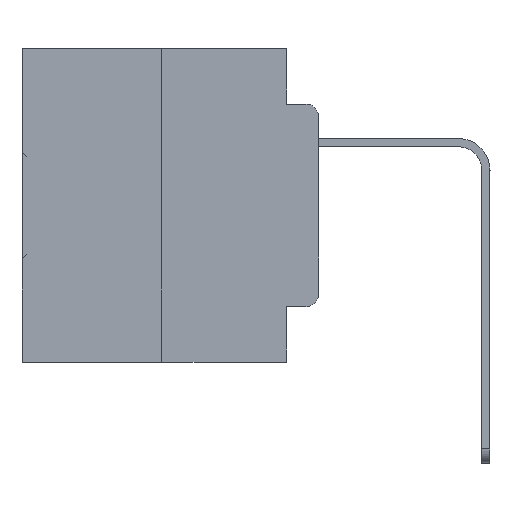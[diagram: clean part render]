
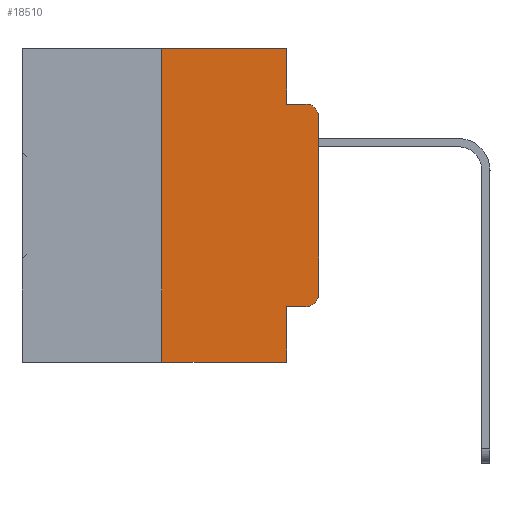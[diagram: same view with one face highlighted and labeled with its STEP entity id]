
A CAD part, left-side view. The second image highlights one B-rep face of the part: STEP entity #18510.
In plain terms, the highlighted planar face has unit normal (-1, 0, 0).
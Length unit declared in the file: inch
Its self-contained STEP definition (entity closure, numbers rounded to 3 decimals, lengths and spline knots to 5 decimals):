
#1222 = CARTESIAN_POINT ( 'NONE',  ( 0., 0.02, -0.3915 ) ) ;
#1315 = VERTEX_POINT ( 'NONE', #25209 ) ;
#1400 = CARTESIAN_POINT ( 'NONE',  ( 0., 0.25, -0.5 ) ) ;
#1501 = ORIENTED_EDGE ( 'NONE', *, *, #22734, .T. ) ;
#1895 = VERTEX_POINT ( 'NONE', #10665 ) ;
#2087 = LINE ( 'NONE', #16711, #18109 ) ;
#2562 = EDGE_CURVE ( 'NONE', #29663, #1315, #13402, .T. ) ;
#2696 = CARTESIAN_POINT ( 'NONE',  ( 0., 0.473, 0. ) ) ;
#4146 = DIRECTION ( 'NONE',  ( 0., 0., -1. ) ) ;
#4202 = ORIENTED_EDGE ( 'NONE', *, *, #4805, .T. ) ;
#4276 = VERTEX_POINT ( 'NONE', #26540 ) ;
#4565 = EDGE_CURVE ( 'NONE', #1895, #23174, #22686, .T. ) ;
#4805 = EDGE_CURVE ( 'NONE', #1895, #22444, #16731, .T. ) ;
#5413 = VERTEX_POINT ( 'NONE', #1400 ) ;
#5430 = PLANE ( 'NONE',  #19464 ) ;
#6024 = DIRECTION ( 'NONE',  ( -1., 0., 0. ) ) ;
#6452 = EDGE_CURVE ( 'NONE', #5413, #23174, #11142, .T. ) ;
#7664 = VERTEX_POINT ( 'NONE', #12583 ) ;
#7718 = DIRECTION ( 'NONE',  ( 0., 0., -1. ) ) ;
#8043 = CARTESIAN_POINT ( 'NONE',  ( 0., 0.473, 0. ) ) ;
#9430 = ORIENTED_EDGE ( 'NONE', *, *, #14590, .F. ) ;
#9458 = CIRCLE ( 'NONE', #17856, 0.02 ) ;
#10326 = DIRECTION ( 'NONE',  ( 1., 0., 0. ) ) ;
#10528 = CARTESIAN_POINT ( 'NONE',  ( 0., 0.051, -0.0885 ) ) ;
#10665 = CARTESIAN_POINT ( 'NONE',  ( 0., 0.051, -0.4115 ) ) ;
#10778 = CARTESIAN_POINT ( 'NONE',  ( 0., 0.02, -0.1085 ) ) ;
#11057 = CIRCLE ( 'NONE', #13010, 0.02 ) ;
#11142 = LINE ( 'NONE', #13102, #27224 ) ;
#11158 = CARTESIAN_POINT ( 'NONE',  ( 0., 0., -0.3915 ) ) ;
#11638 = VECTOR ( 'NONE', #18607, 39.37008 ) ;
#11715 = VERTEX_POINT ( 'NONE', #11158 ) ;
#12320 = CARTESIAN_POINT ( 'NONE',  ( 0., 0.051, -0.5 ) ) ;
#12468 = DIRECTION ( 'NONE',  ( 0., 0., -1. ) ) ;
#12565 = ORIENTED_EDGE ( 'NONE', *, *, #23254, .T. ) ;
#12583 = CARTESIAN_POINT ( 'NONE',  ( 0., 0.02, -0.0885 ) ) ;
#12961 = DIRECTION ( 'NONE',  ( 0., -1., 0. ) ) ;
#13010 = AXIS2_PLACEMENT_3D ( 'NONE', #1222, #6024, #21031 ) ;
#13091 = LINE ( 'NONE', #19133, #31496 ) ;
#13102 = CARTESIAN_POINT ( 'NONE',  ( 0., 0.473, -0.5 ) ) ;
#13402 = LINE ( 'NONE', #2696, #20873 ) ;
#13518 = LINE ( 'NONE', #10528, #14321 ) ;
#14321 = VECTOR ( 'NONE', #17879, 39.37008 ) ;
#14590 = EDGE_CURVE ( 'NONE', #14788, #7664, #13518, .T. ) ;
#14788 = VERTEX_POINT ( 'NONE', #31764 ) ;
#15029 = LINE ( 'NONE', #18474, #27222 ) ;
#15405 = DIRECTION ( 'NONE',  ( 0., -1., 0. ) ) ;
#15421 = ORIENTED_EDGE ( 'NONE', *, *, #4565, .F. ) ;
#15970 = VECTOR ( 'NONE', #12468, 39.37008 ) ;
#16271 = EDGE_LOOP ( 'NONE', ( #18104, #12565, #9430, #29316, #27624, #16427, #31915, #15421, #4202, #1501 ) ) ;
#16427 = ORIENTED_EDGE ( 'NONE', *, *, #27830, .F. ) ;
#16711 = CARTESIAN_POINT ( 'NONE',  ( 0., 0.051, 0. ) ) ;
#16731 = LINE ( 'NONE', #18835, #11638 ) ;
#16801 = DIRECTION ( 'NONE',  ( 0., 0., 1. ) ) ;
#17423 = CARTESIAN_POINT ( 'NONE',  ( 0., 0.25, 0. ) ) ;
#17856 = AXIS2_PLACEMENT_3D ( 'NONE', #10778, #30367, #23298 ) ;
#17879 = DIRECTION ( 'NONE',  ( 0., -1., 0. ) ) ;
#18104 = ORIENTED_EDGE ( 'NONE', *, *, #27972, .T. ) ;
#18109 = VECTOR ( 'NONE', #4146, 39.37008 ) ;
#18234 = FACE_OUTER_BOUND ( 'NONE', #16271, .T. ) ;
#18474 = CARTESIAN_POINT ( 'NONE',  ( 0., 0.25, 0. ) ) ;
#18510 = ADVANCED_FACE ( 'NONE', ( #18234 ), #5430, .F. ) ;
#18607 = DIRECTION ( 'NONE',  ( 0., -1., 0. ) ) ;
#18835 = CARTESIAN_POINT ( 'NONE',  ( 0., 0.051, -0.4115 ) ) ;
#19133 = CARTESIAN_POINT ( 'NONE',  ( 0., 0., 0. ) ) ;
#19464 = AXIS2_PLACEMENT_3D ( 'NONE', #8043, #10326, #7718 ) ;
#20873 = VECTOR ( 'NONE', #12961, 39.37008 ) ;
#21007 = DIRECTION ( 'NONE',  ( 0., 0., 1. ) ) ;
#21031 = DIRECTION ( 'NONE',  ( 0., 0., -1. ) ) ;
#22277 = CARTESIAN_POINT ( 'NONE',  ( 0., 0.02, -0.4115 ) ) ;
#22444 = VERTEX_POINT ( 'NONE', #22277 ) ;
#22686 = LINE ( 'NONE', #30090, #15970 ) ;
#22734 = EDGE_CURVE ( 'NONE', #22444, #11715, #11057, .T. ) ;
#22915 = EDGE_CURVE ( 'NONE', #1315, #14788, #2087, .T. ) ;
#23174 = VERTEX_POINT ( 'NONE', #12320 ) ;
#23254 = EDGE_CURVE ( 'NONE', #4276, #7664, #9458, .T. ) ;
#23298 = DIRECTION ( 'NONE',  ( 0., 0., -1. ) ) ;
#25209 = CARTESIAN_POINT ( 'NONE',  ( 0., 0.051, 0. ) ) ;
#26540 = CARTESIAN_POINT ( 'NONE',  ( 0., 0., -0.1085 ) ) ;
#27222 = VECTOR ( 'NONE', #21007, 39.37008 ) ;
#27224 = VECTOR ( 'NONE', #15405, 39.37008 ) ;
#27624 = ORIENTED_EDGE ( 'NONE', *, *, #2562, .F. ) ;
#27830 = EDGE_CURVE ( 'NONE', #5413, #29663, #15029, .T. ) ;
#27972 = EDGE_CURVE ( 'NONE', #11715, #4276, #13091, .T. ) ;
#29316 = ORIENTED_EDGE ( 'NONE', *, *, #22915, .F. ) ;
#29663 = VERTEX_POINT ( 'NONE', #17423 ) ;
#30090 = CARTESIAN_POINT ( 'NONE',  ( 0., 0.051, 0. ) ) ;
#30367 = DIRECTION ( 'NONE',  ( -1., 0., 0. ) ) ;
#31496 = VECTOR ( 'NONE', #16801, 39.37008 ) ;
#31764 = CARTESIAN_POINT ( 'NONE',  ( 0., 0.051, -0.0885 ) ) ;
#31915 = ORIENTED_EDGE ( 'NONE', *, *, #6452, .T. ) ;
